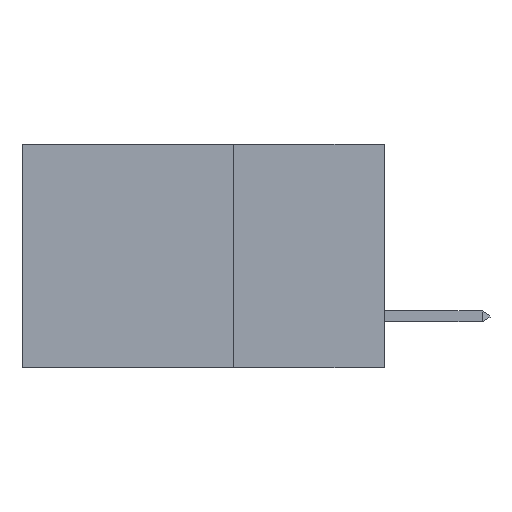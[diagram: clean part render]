
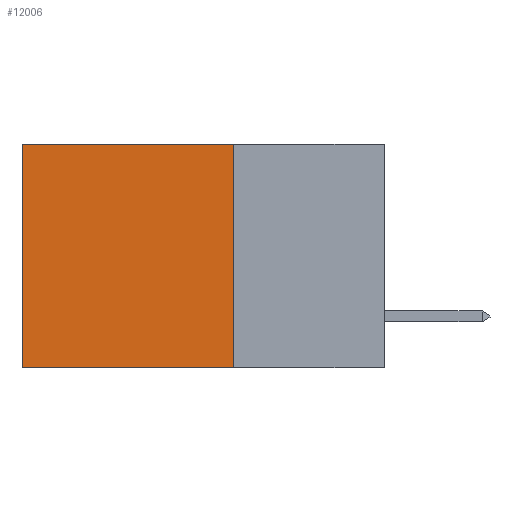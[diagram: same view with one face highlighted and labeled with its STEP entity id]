
A CAD part, left-side view. The second image highlights one B-rep face of the part: STEP entity #12006.
In plain terms, the highlighted planar face has unit normal (-1, 0, 0).
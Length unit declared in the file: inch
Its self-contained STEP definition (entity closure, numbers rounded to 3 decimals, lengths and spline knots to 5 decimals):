
#1032 = CARTESIAN_POINT ( 'NONE',  ( 0.2875, 0.25, -0.37 ) ) ;
#1106 = ORIENTED_EDGE ( 'NONE', *, *, #17258, .F. ) ;
#1922 = EDGE_CURVE ( 'NONE', #19516, #11220, #14163, .T. ) ;
#2610 = LINE ( 'NONE', #8273, #10553 ) ;
#2935 = VERTEX_POINT ( 'NONE', #1032 ) ;
#3556 = VERTEX_POINT ( 'NONE', #19791 ) ;
#4258 = CARTESIAN_POINT ( 'NONE',  ( 0.2875, 0.25, 0. ) ) ;
#4430 = ORIENTED_EDGE ( 'NONE', *, *, #1922, .T. ) ;
#5610 = DIRECTION ( 'NONE',  ( 0., 0., -1. ) ) ;
#6832 = CARTESIAN_POINT ( 'NONE',  ( 0.2875, 0.25, -0.37 ) ) ;
#7958 = CARTESIAN_POINT ( 'NONE',  ( 0.2875, 0.25, 0. ) ) ;
#8273 = CARTESIAN_POINT ( 'NONE',  ( 0.2875, 0.6, 0. ) ) ;
#9340 = EDGE_CURVE ( 'NONE', #11220, #3556, #2610, .T. ) ;
#9657 = FACE_OUTER_BOUND ( 'NONE', #18357, .T. ) ;
#9727 = CARTESIAN_POINT ( 'NONE',  ( 0.2875, 0.6, 0. ) ) ;
#9857 = DIRECTION ( 'NONE',  ( 0., 0., -1. ) ) ;
#10553 = VECTOR ( 'NONE', #9857, 39.37008 ) ;
#11220 = VERTEX_POINT ( 'NONE', #9727 ) ;
#11938 = PLANE ( 'NONE',  #13967 ) ;
#12006 = ADVANCED_FACE ( 'NONE', ( #9657 ), #11938, .F. ) ;
#12348 = VECTOR ( 'NONE', #15775, 39.37008 ) ;
#12801 = ORIENTED_EDGE ( 'NONE', *, *, #9340, .T. ) ;
#12924 = EDGE_CURVE ( 'NONE', #19516, #2935, #17022, .T. ) ;
#12932 = VECTOR ( 'NONE', #19518, 39.37008 ) ;
#13540 = CARTESIAN_POINT ( 'NONE',  ( 0.2875, 0.25, 0. ) ) ;
#13666 = VECTOR ( 'NONE', #18910, 39.37008 ) ;
#13967 = AXIS2_PLACEMENT_3D ( 'NONE', #13540, #15106, #5610 ) ;
#14163 = LINE ( 'NONE', #19048, #13666 ) ;
#15106 = DIRECTION ( 'NONE',  ( 1., 0., 0. ) ) ;
#15775 = DIRECTION ( 'NONE',  ( 0., 0., -1. ) ) ;
#15870 = ORIENTED_EDGE ( 'NONE', *, *, #12924, .F. ) ;
#17022 = LINE ( 'NONE', #7958, #12348 ) ;
#17258 = EDGE_CURVE ( 'NONE', #2935, #3556, #17613, .T. ) ;
#17613 = LINE ( 'NONE', #6832, #12932 ) ;
#18357 = EDGE_LOOP ( 'NONE', ( #12801, #1106, #15870, #4430 ) ) ;
#18910 = DIRECTION ( 'NONE',  ( 0., 1., 0. ) ) ;
#19048 = CARTESIAN_POINT ( 'NONE',  ( 0.2875, 0.25, 0. ) ) ;
#19516 = VERTEX_POINT ( 'NONE', #4258 ) ;
#19518 = DIRECTION ( 'NONE',  ( 0., 1., 0. ) ) ;
#19791 = CARTESIAN_POINT ( 'NONE',  ( 0.2875, 0.6, -0.37 ) ) ;
